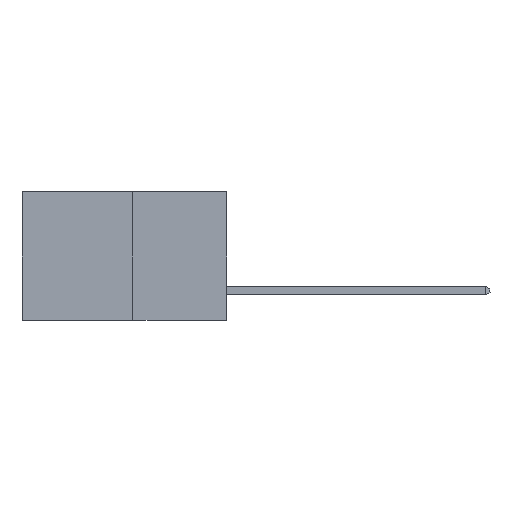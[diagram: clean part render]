
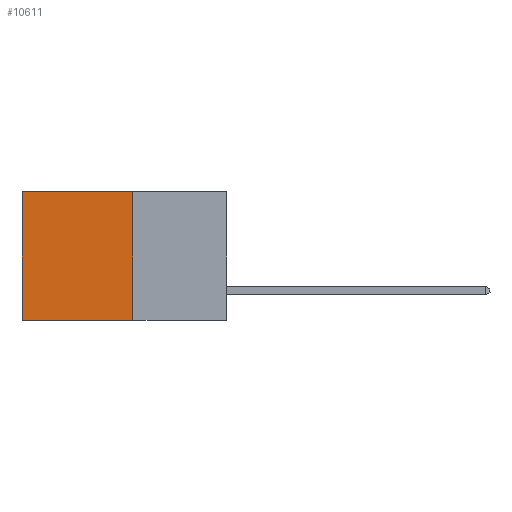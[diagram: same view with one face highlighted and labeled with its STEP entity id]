
A CAD part, left-side view. The second image highlights one B-rep face of the part: STEP entity #10611.
In plain terms, the highlighted planar face has unit normal (-1, 0, 0).
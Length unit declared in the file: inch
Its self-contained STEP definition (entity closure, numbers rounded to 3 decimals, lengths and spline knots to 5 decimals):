
#3 = DIRECTION ( 'NONE',  ( 0., 0., -1. ) ) ;
#109 = EDGE_CURVE ( 'NONE', #782, #10117, #6847, .T. ) ;
#126 = LINE ( 'NONE', #2772, #9240 ) ;
#782 = VERTEX_POINT ( 'NONE', #9891 ) ;
#1347 = EDGE_CURVE ( 'NONE', #7114, #4283, #6426, .T. ) ;
#1799 = CARTESIAN_POINT ( 'NONE',  ( 0.277, 0.59, -0.37 ) ) ;
#2513 = ORIENTED_EDGE ( 'NONE', *, *, #10167, .T. ) ;
#2653 = AXIS2_PLACEMENT_3D ( 'NONE', #8649, #3434, #9463 ) ;
#2772 = CARTESIAN_POINT ( 'NONE',  ( 0.277, 0.59, -0.37 ) ) ;
#3434 = DIRECTION ( 'NONE',  ( 1., 0., 0. ) ) ;
#3753 = EDGE_LOOP ( 'NONE', ( #2513, #4264, #10901, #9790 ) ) ;
#3866 = EDGE_CURVE ( 'NONE', #7114, #782, #4412, .T. ) ;
#4152 = CARTESIAN_POINT ( 'NONE',  ( 0.277, 0.27, 0. ) ) ;
#4264 = ORIENTED_EDGE ( 'NONE', *, *, #109, .F. ) ;
#4283 = VERTEX_POINT ( 'NONE', #10079 ) ;
#4412 = LINE ( 'NONE', #5625, #6475 ) ;
#5625 = CARTESIAN_POINT ( 'NONE',  ( 0.277, 0.27, -0.37 ) ) ;
#6074 = DIRECTION ( 'NONE',  ( 0., 1., 0. ) ) ;
#6426 = LINE ( 'NONE', #4152, #6679 ) ;
#6462 = DIRECTION ( 'NONE',  ( 0., 1., 0. ) ) ;
#6475 = VECTOR ( 'NONE', #10666, 39.37008 ) ;
#6679 = VECTOR ( 'NONE', #6074, 39.37008 ) ;
#6847 = LINE ( 'NONE', #6951, #8887 ) ;
#6951 = CARTESIAN_POINT ( 'NONE',  ( 0.277, 0.27, -0.37 ) ) ;
#7114 = VERTEX_POINT ( 'NONE', #10877 ) ;
#8452 = FACE_OUTER_BOUND ( 'NONE', #3753, .T. ) ;
#8649 = CARTESIAN_POINT ( 'NONE',  ( 0.277, 0.27, -0.37 ) ) ;
#8887 = VECTOR ( 'NONE', #6462, 39.37008 ) ;
#9240 = VECTOR ( 'NONE', #3, 39.37008 ) ;
#9463 = DIRECTION ( 'NONE',  ( 0., 0., -1. ) ) ;
#9790 = ORIENTED_EDGE ( 'NONE', *, *, #1347, .T. ) ;
#9891 = CARTESIAN_POINT ( 'NONE',  ( 0.277, 0.27, -0.37 ) ) ;
#10079 = CARTESIAN_POINT ( 'NONE',  ( 0.277, 0.59, 0. ) ) ;
#10117 = VERTEX_POINT ( 'NONE', #1799 ) ;
#10167 = EDGE_CURVE ( 'NONE', #4283, #10117, #126, .T. ) ;
#10611 = ADVANCED_FACE ( 'NONE', ( #8452 ), #11013, .F. ) ;
#10666 = DIRECTION ( 'NONE',  ( 0., 0., -1. ) ) ;
#10877 = CARTESIAN_POINT ( 'NONE',  ( 0.277, 0.27, 0. ) ) ;
#10901 = ORIENTED_EDGE ( 'NONE', *, *, #3866, .F. ) ;
#11013 = PLANE ( 'NONE',  #2653 ) ;
